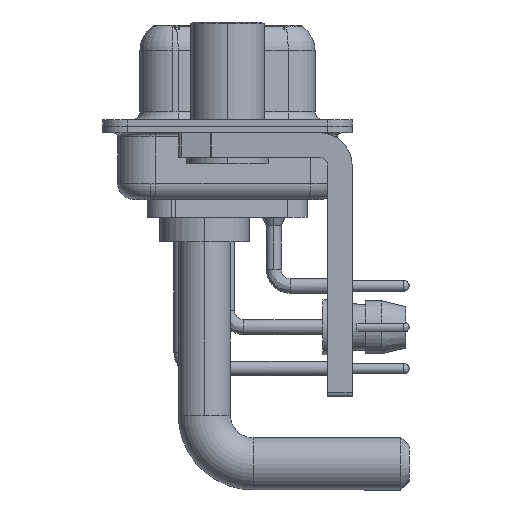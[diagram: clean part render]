
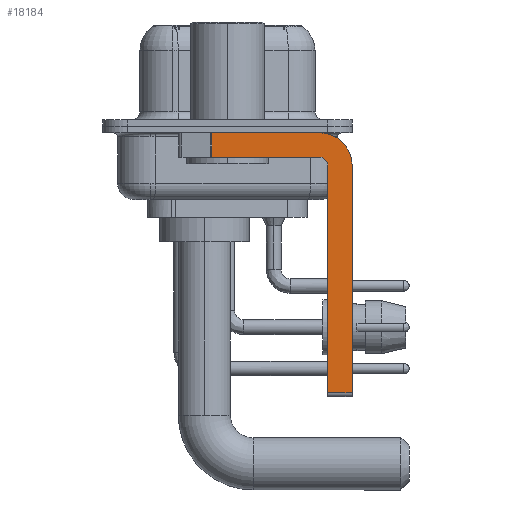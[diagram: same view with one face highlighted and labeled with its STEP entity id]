
A CAD part, left-side view. The second image highlights one B-rep face of the part: STEP entity #18184.
In plain terms, the highlighted planar face has unit normal (-1, 0, 0).
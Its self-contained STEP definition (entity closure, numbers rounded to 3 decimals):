
#1756 = AXIS2_PLACEMENT_3D ( 'NONE', #12779, #2607, #28855 ) ;
#2159 = AXIS2_PLACEMENT_3D ( 'NONE', #9876, #30539, #25139 ) ;
#2607 = DIRECTION ( 'NONE',  ( 1., 0., 0. ) ) ;
#3520 = ORIENTED_EDGE ( 'NONE', *, *, #23382, .F. ) ;
#4675 = ORIENTED_EDGE ( 'NONE', *, *, #22090, .F. ) ;
#4959 = PLANE ( 'NONE',  #2159 ) ;
#5739 = DIRECTION ( 'NONE',  ( 0., -1., 0. ) ) ;
#6395 = EDGE_CURVE ( 'NONE', #19269, #13983, #13949, .T. ) ;
#6730 = EDGE_CURVE ( 'NONE', #30612, #14812, #15282, .T. ) ;
#6983 = ORIENTED_EDGE ( 'NONE', *, *, #22114, .F. ) ;
#7583 = ORIENTED_EDGE ( 'NONE', *, *, #26248, .T. ) ;
#7757 = CARTESIAN_POINT ( 'NONE',  ( -2.9, 3., -0.4 ) ) ;
#7820 = VECTOR ( 'NONE', #5739, 1000. ) ;
#8011 = DIRECTION ( 'NONE',  ( 0., -1., 0. ) ) ;
#8402 = CARTESIAN_POINT ( 'NONE',  ( -2.9, -6.15, -16.35 ) ) ;
#8647 = VERTEX_POINT ( 'NONE', #26333 ) ;
#9229 = VECTOR ( 'NONE', #10198, 1000. ) ;
#9876 = CARTESIAN_POINT ( 'NONE',  ( -2.9, -5.65, -2.4 ) ) ;
#10149 = VERTEX_POINT ( 'NONE', #11919 ) ;
#10198 = DIRECTION ( 'NONE',  ( 0., 0., -1. ) ) ;
#10354 = DIRECTION ( 'NONE',  ( 0., 0., 1. ) ) ;
#10457 = VECTOR ( 'NONE', #13189, 1000. ) ;
#10566 = CARTESIAN_POINT ( 'NONE',  ( -2.9, -5.65, -16.35 ) ) ;
#11582 = AXIS2_PLACEMENT_3D ( 'NONE', #15757, #21015, #10354 ) ;
#11695 = CARTESIAN_POINT ( 'NONE',  ( -2.9, 0.978, -0.4 ) ) ;
#11919 = CARTESIAN_POINT ( 'NONE',  ( -2.9, -5.65, -1.9 ) ) ;
#12674 = CARTESIAN_POINT ( 'NONE',  ( -2.9, 0.978, -1.9 ) ) ;
#12779 = CARTESIAN_POINT ( 'NONE',  ( -2.9, -5.65, -2.4 ) ) ;
#13189 = DIRECTION ( 'NONE',  ( 0., 1., 0. ) ) ;
#13484 = CARTESIAN_POINT ( 'NONE',  ( -2.9, -7.65, -2.4 ) ) ;
#13949 = LINE ( 'NONE', #29205, #32492 ) ;
#13983 = VERTEX_POINT ( 'NONE', #17879 ) ;
#14812 = VERTEX_POINT ( 'NONE', #12674 ) ;
#15177 = ORIENTED_EDGE ( 'NONE', *, *, #24531, .F. ) ;
#15282 = LINE ( 'NONE', #28009, #9229 ) ;
#15344 = ORIENTED_EDGE ( 'NONE', *, *, #6395, .F. ) ;
#15404 = LINE ( 'NONE', #25767, #10457 ) ;
#15563 = LINE ( 'NONE', #7757, #7820 ) ;
#15757 = CARTESIAN_POINT ( 'NONE',  ( -2.9, -5.65, -2.4 ) ) ;
#15898 = CIRCLE ( 'NONE', #11582, 0.5 ) ;
#15968 = CARTESIAN_POINT ( 'NONE',  ( -2.9, -6.15, -16.6 ) ) ;
#16562 = ORIENTED_EDGE ( 'NONE', *, *, #6730, .T. ) ;
#17879 = CARTESIAN_POINT ( 'NONE',  ( -2.9, -7.65, -16.35 ) ) ;
#18184 = ADVANCED_FACE ( 'NONE', ( #20040 ), #4959, .F. ) ;
#19269 = VERTEX_POINT ( 'NONE', #13484 ) ;
#20040 = FACE_OUTER_BOUND ( 'NONE', #23194, .T. ) ;
#20651 = VERTEX_POINT ( 'NONE', #8402 ) ;
#21015 = DIRECTION ( 'NONE',  ( -1., 0., 0. ) ) ;
#21886 = CARTESIAN_POINT ( 'NONE',  ( -2.9, -5.65, -0.4 ) ) ;
#22090 = EDGE_CURVE ( 'NONE', #31687, #19269, #22865, .T. ) ;
#22114 = EDGE_CURVE ( 'NONE', #20651, #8647, #23623, .T. ) ;
#22865 = CIRCLE ( 'NONE', #1756, 2. ) ;
#23164 = DIRECTION ( 'NONE',  ( 0., 0., -1. ) ) ;
#23194 = EDGE_LOOP ( 'NONE', ( #32589, #16562, #3520, #15177, #6983, #7583, #15344, #4675 ) ) ;
#23287 = DIRECTION ( 'NONE',  ( 0., 0., 1. ) ) ;
#23382 = EDGE_CURVE ( 'NONE', #10149, #14812, #15404, .T. ) ;
#23623 = LINE ( 'NONE', #15968, #27195 ) ;
#24531 = EDGE_CURVE ( 'NONE', #8647, #10149, #15898, .T. ) ;
#24689 = VECTOR ( 'NONE', #8011, 1000. ) ;
#25139 = DIRECTION ( 'NONE',  ( 0., 0., -1. ) ) ;
#25264 = EDGE_CURVE ( 'NONE', #30612, #31687, #15563, .T. ) ;
#25767 = CARTESIAN_POINT ( 'NONE',  ( -2.9, -5.65, -1.9 ) ) ;
#26248 = EDGE_CURVE ( 'NONE', #20651, #13983, #28694, .T. ) ;
#26333 = CARTESIAN_POINT ( 'NONE',  ( -2.9, -6.15, -2.4 ) ) ;
#27195 = VECTOR ( 'NONE', #23287, 1000. ) ;
#28009 = CARTESIAN_POINT ( 'NONE',  ( -2.9, 0.978, -1.9 ) ) ;
#28694 = LINE ( 'NONE', #10566, #24689 ) ;
#28855 = DIRECTION ( 'NONE',  ( 0., 0., -1. ) ) ;
#29205 = CARTESIAN_POINT ( 'NONE',  ( -2.9, -7.65, -2.4 ) ) ;
#30539 = DIRECTION ( 'NONE',  ( 1., 0., 0. ) ) ;
#30612 = VERTEX_POINT ( 'NONE', #11695 ) ;
#31687 = VERTEX_POINT ( 'NONE', #21886 ) ;
#32492 = VECTOR ( 'NONE', #23164, 1000. ) ;
#32589 = ORIENTED_EDGE ( 'NONE', *, *, #25264, .F. ) ;
